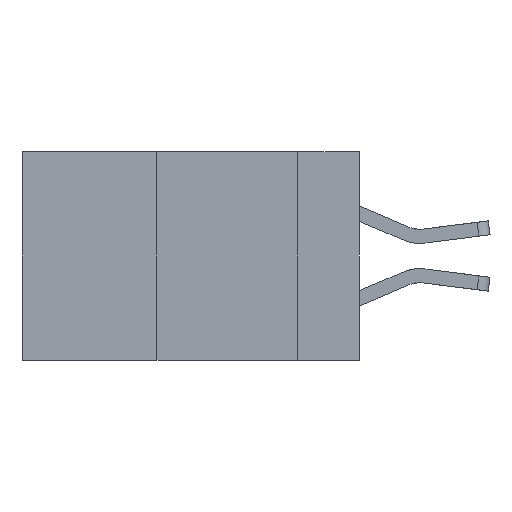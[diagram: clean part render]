
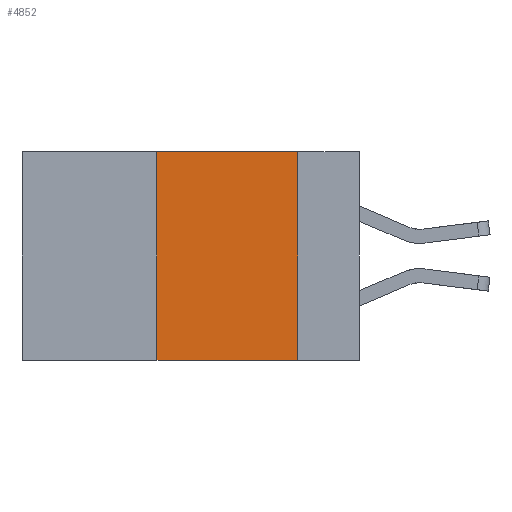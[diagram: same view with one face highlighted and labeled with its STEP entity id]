
A CAD part, left-side view. The second image highlights one B-rep face of the part: STEP entity #4852.
In plain terms, the highlighted planar face has unit normal (-1, 0, 0).
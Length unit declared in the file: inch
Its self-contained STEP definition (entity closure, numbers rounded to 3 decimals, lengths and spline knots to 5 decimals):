
#360 = CARTESIAN_POINT ( 'NONE',  ( 0., 0.36, 0. ) ) ;
#572 = VECTOR ( 'NONE', #4793, 39.37008 ) ;
#839 = CARTESIAN_POINT ( 'NONE',  ( 0., 0.6, 0. ) ) ;
#1151 = EDGE_CURVE ( 'NONE', #4980, #11999, #1647, .T. ) ;
#1545 = EDGE_CURVE ( 'NONE', #6636, #6660, #5918, .T. ) ;
#1647 = LINE ( 'NONE', #3951, #3308 ) ;
#1811 = LINE ( 'NONE', #4850, #12329 ) ;
#2181 = DIRECTION ( 'NONE',  ( 0., 0., 1. ) ) ;
#2298 = DIRECTION ( 'NONE',  ( 0., 0., -1. ) ) ;
#3308 = VECTOR ( 'NONE', #10766, 39.37008 ) ;
#3374 = CARTESIAN_POINT ( 'NONE',  ( 0., 0.11, -0.37 ) ) ;
#3377 = ORIENTED_EDGE ( 'NONE', *, *, #1151, .T. ) ;
#3476 = FACE_OUTER_BOUND ( 'NONE', #4091, .T. ) ;
#3951 = CARTESIAN_POINT ( 'NONE',  ( 0., 0.6, -0.37 ) ) ;
#4091 = EDGE_LOOP ( 'NONE', ( #7830, #10023, #5650, #3377 ) ) ;
#4583 = CARTESIAN_POINT ( 'NONE',  ( 0., 0.11, 0. ) ) ;
#4793 = DIRECTION ( 'NONE',  ( 0., -1., 0. ) ) ;
#4850 = CARTESIAN_POINT ( 'NONE',  ( 0., 0.11, 0. ) ) ;
#4852 = ADVANCED_FACE ( 'NONE', ( #3476 ), #12262, .F. ) ;
#4908 = DIRECTION ( 'NONE',  ( 0., 0., -1. ) ) ;
#4980 = VERTEX_POINT ( 'NONE', #9755 ) ;
#5215 = LINE ( 'NONE', #5946, #10850 ) ;
#5650 = ORIENTED_EDGE ( 'NONE', *, *, #8154, .F. ) ;
#5918 = LINE ( 'NONE', #839, #572 ) ;
#5946 = CARTESIAN_POINT ( 'NONE',  ( 0., 0.36, 0. ) ) ;
#6636 = VERTEX_POINT ( 'NONE', #360 ) ;
#6660 = VERTEX_POINT ( 'NONE', #4583 ) ;
#7830 = ORIENTED_EDGE ( 'NONE', *, *, #8832, .F. ) ;
#8154 = EDGE_CURVE ( 'NONE', #4980, #6636, #5215, .T. ) ;
#8437 = CARTESIAN_POINT ( 'NONE',  ( 0., 0.6, 0. ) ) ;
#8832 = EDGE_CURVE ( 'NONE', #6660, #11999, #1811, .T. ) ;
#9498 = DIRECTION ( 'NONE',  ( 1., 0., 0. ) ) ;
#9755 = CARTESIAN_POINT ( 'NONE',  ( 0., 0.36, -0.37 ) ) ;
#10023 = ORIENTED_EDGE ( 'NONE', *, *, #1545, .F. ) ;
#10766 = DIRECTION ( 'NONE',  ( 0., -1., 0. ) ) ;
#10850 = VECTOR ( 'NONE', #2181, 39.37008 ) ;
#11999 = VERTEX_POINT ( 'NONE', #3374 ) ;
#12262 = PLANE ( 'NONE',  #12833 ) ;
#12329 = VECTOR ( 'NONE', #4908, 39.37008 ) ;
#12833 = AXIS2_PLACEMENT_3D ( 'NONE', #8437, #9498, #2298 ) ;
